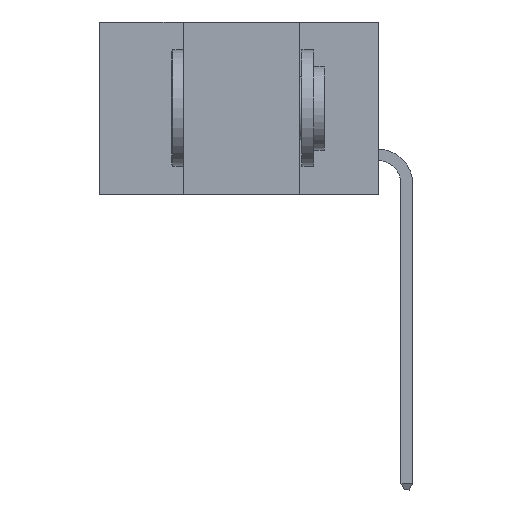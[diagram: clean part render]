
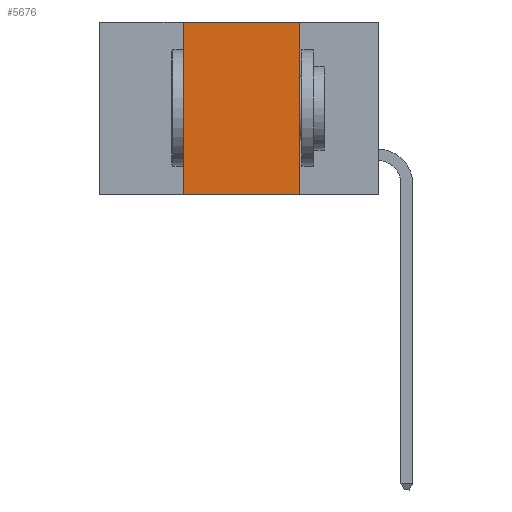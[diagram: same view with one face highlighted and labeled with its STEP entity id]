
A CAD part, left-side view. The second image highlights one B-rep face of the part: STEP entity #5676.
In plain terms, the highlighted planar face has unit normal (-1, 0, 0).
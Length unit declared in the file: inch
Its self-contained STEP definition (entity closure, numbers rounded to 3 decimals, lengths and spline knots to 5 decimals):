
#330 = CARTESIAN_POINT ( 'NONE',  ( 0., 0.6, 0. ) ) ;
#348 = CARTESIAN_POINT ( 'NONE',  ( 0., 0.6, -0.37 ) ) ;
#856 = LINE ( 'NONE', #9030, #16336 ) ;
#1002 = VERTEX_POINT ( 'NONE', #2217 ) ;
#2217 = CARTESIAN_POINT ( 'NONE',  ( 0., 0.42, -0.37 ) ) ;
#2928 = CARTESIAN_POINT ( 'NONE',  ( 0., 0.17, -0.37 ) ) ;
#4007 = EDGE_CURVE ( 'NONE', #1002, #16196, #12750, .T. ) ;
#4774 = VECTOR ( 'NONE', #13310, 39.37008 ) ;
#5197 = DIRECTION ( 'NONE',  ( 0., 0., -1. ) ) ;
#5676 = ADVANCED_FACE ( 'NONE', ( #10208 ), #8587, .F. ) ;
#5872 = DIRECTION ( 'NONE',  ( 1., 0., 0. ) ) ;
#6778 = ORIENTED_EDGE ( 'NONE', *, *, #16475, .F. ) ;
#7955 = EDGE_CURVE ( 'NONE', #9594, #16196, #10618, .T. ) ;
#8587 = PLANE ( 'NONE',  #15263 ) ;
#9030 = CARTESIAN_POINT ( 'NONE',  ( 0., 0.6, 0. ) ) ;
#9082 = LINE ( 'NONE', #17555, #4774 ) ;
#9459 = CARTESIAN_POINT ( 'NONE',  ( 0., 0.17, -0.37 ) ) ;
#9594 = VERTEX_POINT ( 'NONE', #13210 ) ;
#9793 = ORIENTED_EDGE ( 'NONE', *, *, #15471, .F. ) ;
#10208 = FACE_OUTER_BOUND ( 'NONE', #14411, .T. ) ;
#10618 = LINE ( 'NONE', #9459, #11277 ) ;
#11277 = VECTOR ( 'NONE', #5197, 39.37008 ) ;
#11381 = DIRECTION ( 'NONE',  ( 0., -1., 0. ) ) ;
#11847 = CARTESIAN_POINT ( 'NONE',  ( 0., 0.42, 0. ) ) ;
#12750 = LINE ( 'NONE', #348, #16614 ) ;
#12816 = DIRECTION ( 'NONE',  ( 0., 0., -1. ) ) ;
#12985 = DIRECTION ( 'NONE',  ( 0., -1., 0. ) ) ;
#13186 = ORIENTED_EDGE ( 'NONE', *, *, #7955, .F. ) ;
#13210 = CARTESIAN_POINT ( 'NONE',  ( 0., 0.17, 0. ) ) ;
#13310 = DIRECTION ( 'NONE',  ( 0., 0., 1. ) ) ;
#13756 = VERTEX_POINT ( 'NONE', #11847 ) ;
#14411 = EDGE_LOOP ( 'NONE', ( #13186, #9793, #6778, #15625 ) ) ;
#15263 = AXIS2_PLACEMENT_3D ( 'NONE', #330, #5872, #12816 ) ;
#15471 = EDGE_CURVE ( 'NONE', #13756, #9594, #856, .T. ) ;
#15625 = ORIENTED_EDGE ( 'NONE', *, *, #4007, .T. ) ;
#16196 = VERTEX_POINT ( 'NONE', #2928 ) ;
#16336 = VECTOR ( 'NONE', #12985, 39.37008 ) ;
#16475 = EDGE_CURVE ( 'NONE', #1002, #13756, #9082, .T. ) ;
#16614 = VECTOR ( 'NONE', #11381, 39.37008 ) ;
#17555 = CARTESIAN_POINT ( 'NONE',  ( 0., 0.42, -0.37 ) ) ;
